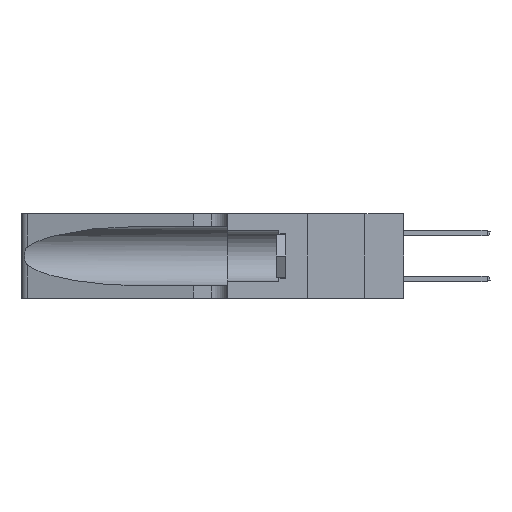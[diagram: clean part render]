
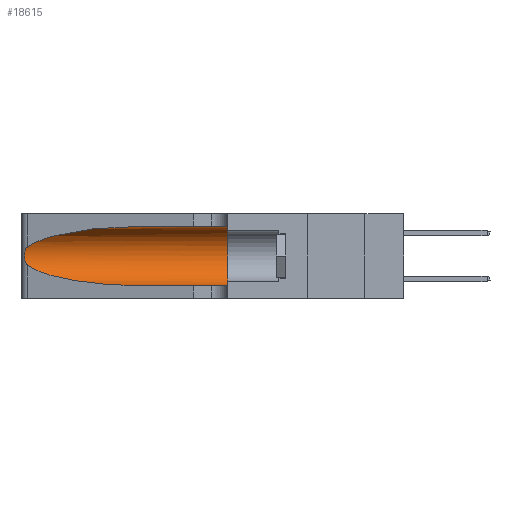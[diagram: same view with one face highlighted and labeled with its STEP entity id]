
A CAD part, left-side view. The second image highlights one B-rep face of the part: STEP entity #18615.
In plain terms, the highlighted cylindrical face has radius 3.308 mm (diameter 6.617 mm), a partial arc.
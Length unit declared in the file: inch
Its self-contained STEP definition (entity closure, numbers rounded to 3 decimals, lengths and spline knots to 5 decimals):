
#447 = CARTESIAN_POINT ( 'NONE',  ( 0.1305, 0.72297, 0.05475 ) ) ;
#579 = ORIENTED_EDGE ( 'NONE', *, *, #33771, .T. ) ;
#590 = CARTESIAN_POINT ( 'NONE',  ( 0.1305, 1.61858, 0.185 ) ) ;
#1255 = B_SPLINE_CURVE_WITH_KNOTS ( 'NONE', 3,
 ( #28743, #26055, #31426, #15278, #34114, #18046, #1525, #20785, #4366, #23465, #7187, #26167, #9954, #28860 ),
 .UNSPECIFIED., .F., .F.,
 ( 4, 2, 2, 2, 2, 2, 4 ),
 ( 0., 0.00027, 0.00053, 0.00107, 0.0016, 0.00187, 0.00214 ),
 .UNSPECIFIED. ) ;
#1273 = VERTEX_POINT ( 'NONE', #6817 ) ;
#1354 = EDGE_CURVE ( 'NONE', #1273, #7210, #1255, .T. ) ;
#1525 = CARTESIAN_POINT ( 'NONE',  ( 0.26075, 1.23896, 0.19203 ) ) ;
#3008 = VECTOR ( 'NONE', #22905, 39.37008 ) ;
#3885 = LINE ( 'NONE', #20221, #3008 ) ;
#4366 = CARTESIAN_POINT ( 'NONE',  ( 0.26017, 1.23833, 0.17102 ) ) ;
#4651 = VERTEX_POINT ( 'NONE', #19641 ) ;
#6817 = CARTESIAN_POINT ( 'NONE',  ( 0.25487, 1.22718, 0.22369 ) ) ;
#7187 = CARTESIAN_POINT ( 'NONE',  ( 0.25789, 1.23486, 0.15765 ) ) ;
#7210 = VERTEX_POINT ( 'NONE', #24153 ) ;
#8548 = VECTOR ( 'NONE', #26779, 39.37008 ) ;
#8904 =( BOUNDED_CURVE ( )  B_SPLINE_CURVE ( 3, ( #11917, #30782, #14648, #33461 ),
 .UNSPECIFIED., .F., .F. ) 
 B_SPLINE_CURVE_WITH_KNOTS ( ( 4, 4 ),
 ( 3.44316, 4.71239 ),
 .UNSPECIFIED. ) 
 CURVE ( )  GEOMETRIC_REPRESENTATION_ITEM ( )  RATIONAL_B_SPLINE_CURVE ( ( 1., 0.87, 0.87, 1. ) ) 
 REPRESENTATION_ITEM ( '' )  );
#8941 = DIRECTION ( 'NONE',  ( 0., 0., -1. ) ) ;
#9411 = LINE ( 'NONE', #24055, #8548 ) ;
#9415 = CYLINDRICAL_SURFACE ( 'NONE', #34254, 0.13025 ) ;
#9954 = CARTESIAN_POINT ( 'NONE',  ( 0.25555, 1.22993, 0.14849 ) ) ;
#10015 = ORIENTED_EDGE ( 'NONE', *, *, #1354, .T. ) ;
#11917 = CARTESIAN_POINT ( 'NONE',  ( 0.25487, 1.22718, 0.14631 ) ) ;
#12719 = DIRECTION ( 'NONE',  ( 0., 1., 0. ) ) ;
#14648 = CARTESIAN_POINT ( 'NONE',  ( 0.18966, 0.96281, 0.05475 ) ) ;
#14666 = EDGE_CURVE ( 'NONE', #18458, #29626, #3885, .T. ) ;
#15278 = CARTESIAN_POINT ( 'NONE',  ( 0.25787, 1.23484, 0.2124 ) ) ;
#15293 = ORIENTED_EDGE ( 'NONE', *, *, #16864, .F. ) ;
#16544 = CARTESIAN_POINT ( 'NONE',  ( 0.18966, 0.96281, 0.31525 ) ) ;
#16666 = CARTESIAN_POINT ( 'NONE',  ( 0.25487, 1.22718, 0.22369 ) ) ;
#16864 = EDGE_CURVE ( 'NONE', #29626, #4651, #30208, .T. ) ;
#18046 = CARTESIAN_POINT ( 'NONE',  ( 0.26018, 1.23835, 0.19895 ) ) ;
#18458 = VERTEX_POINT ( 'NONE', #27296 ) ;
#18615 = ADVANCED_FACE ( 'NONE', ( #31793 ), #9415, .F. ) ;
#19641 = CARTESIAN_POINT ( 'NONE',  ( 0.1305, 0.35, 0.05475 ) ) ;
#19904 = DIRECTION ( 'NONE',  ( 0., -1., 0. ) ) ;
#19923 = EDGE_LOOP ( 'NONE', ( #31092, #10015, #25206, #579, #15293, #28434 ) ) ;
#20221 = CARTESIAN_POINT ( 'NONE',  ( 0.1305, 1.61858, 0.31525 ) ) ;
#20785 = CARTESIAN_POINT ( 'NONE',  ( 0.26075, 1.23896, 0.178 ) ) ;
#21384 = VERTEX_POINT ( 'NONE', #447 ) ;
#22008 = CARTESIAN_POINT ( 'NONE',  ( 0.1305, 0.72297, 0.31525 ) ) ;
#22905 = DIRECTION ( 'NONE',  ( 0., -1., 0. ) ) ;
#23465 = CARTESIAN_POINT ( 'NONE',  ( 0.25856, 1.23593, 0.16098 ) ) ;
#24055 = CARTESIAN_POINT ( 'NONE',  ( 0.1305, 1.61858, 0.05475 ) ) ;
#24153 = CARTESIAN_POINT ( 'NONE',  ( 0.25487, 1.22718, 0.14631 ) ) ;
#25206 = ORIENTED_EDGE ( 'NONE', *, *, #28015, .T. ) ;
#26055 = CARTESIAN_POINT ( 'NONE',  ( 0.25555, 1.22994, 0.2215 ) ) ;
#26167 = CARTESIAN_POINT ( 'NONE',  ( 0.25639, 1.23186, 0.15144 ) ) ;
#26355 = AXIS2_PLACEMENT_3D ( 'NONE', #28898, #12719, #31586 ) ;
#26779 = DIRECTION ( 'NONE',  ( 0., -1., 0. ) ) ;
#27296 = CARTESIAN_POINT ( 'NONE',  ( 0.1305, 0.72297, 0.31525 ) ) ;
#28015 = EDGE_CURVE ( 'NONE', #7210, #21384, #8904, .T. ) ;
#28434 = ORIENTED_EDGE ( 'NONE', *, *, #14666, .F. ) ;
#28743 = CARTESIAN_POINT ( 'NONE',  ( 0.25487, 1.22718, 0.22369 ) ) ;
#28860 = CARTESIAN_POINT ( 'NONE',  ( 0.25487, 1.22718, 0.14631 ) ) ;
#28898 = CARTESIAN_POINT ( 'NONE',  ( 0.1305, 0.35, 0.185 ) ) ;
#29626 = VERTEX_POINT ( 'NONE', #34154 ) ;
#30208 = CIRCLE ( 'NONE', #26355, 0.13025 ) ;
#30782 = CARTESIAN_POINT ( 'NONE',  ( 0.2373, 1.15595, 0.08982 ) ) ;
#31092 = ORIENTED_EDGE ( 'NONE', *, *, #33273, .T. ) ;
#31396 =( BOUNDED_CURVE ( )  B_SPLINE_CURVE ( 3, ( #22008, #16544, #32769, #16666 ),
 .UNSPECIFIED., .F., .F. ) 
 B_SPLINE_CURVE_WITH_KNOTS ( ( 4, 4 ),
 ( 1.5708, 2.84003 ),
 .UNSPECIFIED. ) 
 CURVE ( )  GEOMETRIC_REPRESENTATION_ITEM ( )  RATIONAL_B_SPLINE_CURVE ( ( 1., 0.87, 0.87, 1. ) ) 
 REPRESENTATION_ITEM ( '' )  );
#31426 = CARTESIAN_POINT ( 'NONE',  ( 0.25639, 1.23184, 0.21858 ) ) ;
#31586 = DIRECTION ( 'NONE',  ( 0., 0., 1. ) ) ;
#31793 = FACE_OUTER_BOUND ( 'NONE', #19923, .T. ) ;
#32769 = CARTESIAN_POINT ( 'NONE',  ( 0.2373, 1.15595, 0.28018 ) ) ;
#33273 = EDGE_CURVE ( 'NONE', #18458, #1273, #31396, .T. ) ;
#33461 = CARTESIAN_POINT ( 'NONE',  ( 0.1305, 0.72297, 0.05475 ) ) ;
#33771 = EDGE_CURVE ( 'NONE', #21384, #4651, #9411, .T. ) ;
#34114 = CARTESIAN_POINT ( 'NONE',  ( 0.25854, 1.2359, 0.20912 ) ) ;
#34154 = CARTESIAN_POINT ( 'NONE',  ( 0.1305, 0.35, 0.31525 ) ) ;
#34254 = AXIS2_PLACEMENT_3D ( 'NONE', #590, #19904, #8941 ) ;
